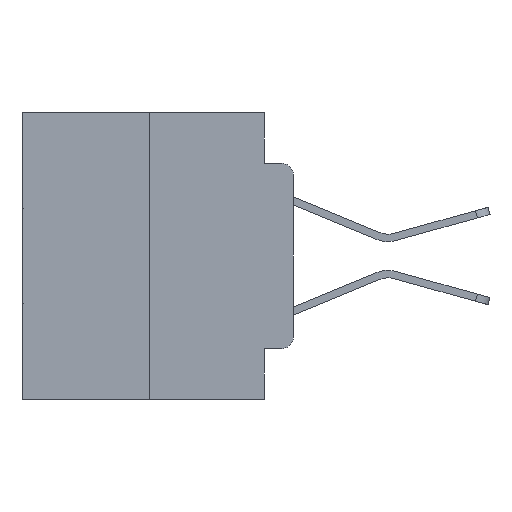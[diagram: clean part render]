
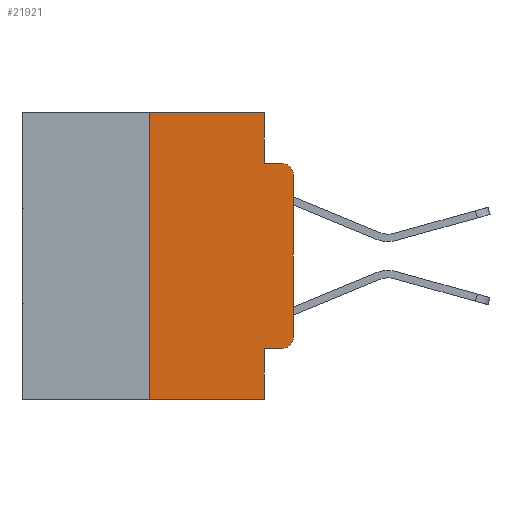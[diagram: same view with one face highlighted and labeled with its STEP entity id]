
A CAD part, left-side view. The second image highlights one B-rep face of the part: STEP entity #21921.
In plain terms, the highlighted planar face has unit normal (-1, 0, 0).
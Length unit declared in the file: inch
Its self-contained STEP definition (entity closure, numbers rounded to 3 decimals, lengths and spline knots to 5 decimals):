
#330 = CARTESIAN_POINT ( 'NONE',  ( 0., 0., -0.1085 ) ) ;
#350 = VECTOR ( 'NONE', #12200, 39.37008 ) ;
#386 = DIRECTION ( 'NONE',  ( 0., 0., -1. ) ) ;
#1704 = DIRECTION ( 'NONE',  ( 0., 0., -1. ) ) ;
#1773 = VECTOR ( 'NONE', #19483, 39.37008 ) ;
#2817 = EDGE_CURVE ( 'NONE', #12098, #9315, #23318, .T. ) ;
#2870 = CARTESIAN_POINT ( 'NONE',  ( 0., 0.473, 0. ) ) ;
#3763 = VECTOR ( 'NONE', #8072, 39.37008 ) ;
#4095 = VERTEX_POINT ( 'NONE', #23252 ) ;
#4832 = ORIENTED_EDGE ( 'NONE', *, *, #26236, .F. ) ;
#4875 = VERTEX_POINT ( 'NONE', #330 ) ;
#5567 = VECTOR ( 'NONE', #23165, 39.37008 ) ;
#5575 = ORIENTED_EDGE ( 'NONE', *, *, #23562, .F. ) ;
#5622 = ORIENTED_EDGE ( 'NONE', *, *, #11684, .T. ) ;
#5971 = DIRECTION ( 'NONE',  ( -1., 0., 0. ) ) ;
#6071 = EDGE_CURVE ( 'NONE', #4095, #27044, #8423, .T. ) ;
#6340 = DIRECTION ( 'NONE',  ( -1., 0., 0. ) ) ;
#6938 = ORIENTED_EDGE ( 'NONE', *, *, #9212, .T. ) ;
#7128 = VERTEX_POINT ( 'NONE', #18365 ) ;
#7258 = CIRCLE ( 'NONE', #7413, 0.02 ) ;
#7413 = AXIS2_PLACEMENT_3D ( 'NONE', #18805, #5971, #20948 ) ;
#8037 = CARTESIAN_POINT ( 'NONE',  ( 0., 0.051, -0.0885 ) ) ;
#8072 = DIRECTION ( 'NONE',  ( 0., -1., 0. ) ) ;
#8423 = LINE ( 'NONE', #21284, #12117 ) ;
#9212 = EDGE_CURVE ( 'NONE', #4875, #13563, #7258, .T. ) ;
#9315 = VERTEX_POINT ( 'NONE', #27440 ) ;
#10048 = CARTESIAN_POINT ( 'NONE',  ( 0., 0.051, -0.4115 ) ) ;
#10429 = CARTESIAN_POINT ( 'NONE',  ( 0., 0.02, -0.0885 ) ) ;
#10655 = ORIENTED_EDGE ( 'NONE', *, *, #6071, .T. ) ;
#11000 = VECTOR ( 'NONE', #13348, 39.37008 ) ;
#11150 = EDGE_CURVE ( 'NONE', #7128, #21916, #21024, .T. ) ;
#11209 = CARTESIAN_POINT ( 'NONE',  ( 0., 0.051, 0. ) ) ;
#11324 = ORIENTED_EDGE ( 'NONE', *, *, #2817, .F. ) ;
#11397 = AXIS2_PLACEMENT_3D ( 'NONE', #19163, #6340, #21306 ) ;
#11595 = CARTESIAN_POINT ( 'NONE',  ( 0., 0.051, -0.4115 ) ) ;
#11684 = EDGE_CURVE ( 'NONE', #21916, #4875, #11994, .T. ) ;
#11979 = LINE ( 'NONE', #26219, #22616 ) ;
#11994 = LINE ( 'NONE', #25247, #5567 ) ;
#12042 = VECTOR ( 'NONE', #20514, 39.37008 ) ;
#12098 = VERTEX_POINT ( 'NONE', #26569 ) ;
#12117 = VECTOR ( 'NONE', #17084, 39.37008 ) ;
#12138 = LINE ( 'NONE', #10048, #350 ) ;
#12200 = DIRECTION ( 'NONE',  ( 0., -1., 0. ) ) ;
#12655 = PLANE ( 'NONE',  #14990 ) ;
#13348 = DIRECTION ( 'NONE',  ( 0., 0., -1. ) ) ;
#13563 = VERTEX_POINT ( 'NONE', #10429 ) ;
#13980 = CARTESIAN_POINT ( 'NONE',  ( 0., 0.051, -0.5 ) ) ;
#14808 = DIRECTION ( 'NONE',  ( 1., 0., 0. ) ) ;
#14983 = ORIENTED_EDGE ( 'NONE', *, *, #20941, .F. ) ;
#14990 = AXIS2_PLACEMENT_3D ( 'NONE', #27368, #14808, #1704 ) ;
#15281 = LINE ( 'NONE', #20758, #3763 ) ;
#15323 = CARTESIAN_POINT ( 'NONE',  ( 0., 0.25, 0. ) ) ;
#17084 = DIRECTION ( 'NONE',  ( 0., -1., 0. ) ) ;
#17808 = VERTEX_POINT ( 'NONE', #8037 ) ;
#17860 = EDGE_LOOP ( 'NONE', ( #5622, #6938, #18990, #5575, #11324, #4832, #10655, #14983, #26830, #19284 ) ) ;
#18365 = CARTESIAN_POINT ( 'NONE',  ( 0., 0.02, -0.4115 ) ) ;
#18805 = CARTESIAN_POINT ( 'NONE',  ( 0., 0.02, -0.1085 ) ) ;
#18939 = EDGE_CURVE ( 'NONE', #26386, #7128, #12138, .T. ) ;
#18990 = ORIENTED_EDGE ( 'NONE', *, *, #23858, .F. ) ;
#19163 = CARTESIAN_POINT ( 'NONE',  ( 0., 0.02, -0.3915 ) ) ;
#19284 = ORIENTED_EDGE ( 'NONE', *, *, #11150, .T. ) ;
#19483 = DIRECTION ( 'NONE',  ( 0., 0., 1. ) ) ;
#20514 = DIRECTION ( 'NONE',  ( 0., -1., 0. ) ) ;
#20758 = CARTESIAN_POINT ( 'NONE',  ( 0., 0.051, -0.0885 ) ) ;
#20941 = EDGE_CURVE ( 'NONE', #26386, #27044, #27762, .T. ) ;
#20948 = DIRECTION ( 'NONE',  ( 0., 0., -1. ) ) ;
#21024 = CIRCLE ( 'NONE', #11397, 0.02 ) ;
#21284 = CARTESIAN_POINT ( 'NONE',  ( 0., 0.473, -0.5 ) ) ;
#21306 = DIRECTION ( 'NONE',  ( 0., 0., -1. ) ) ;
#21916 = VERTEX_POINT ( 'NONE', #25248 ) ;
#21921 = ADVANCED_FACE ( 'NONE', ( #25813 ), #12655, .F. ) ;
#22616 = VECTOR ( 'NONE', #386, 39.37008 ) ;
#23165 = DIRECTION ( 'NONE',  ( 0., 0., 1. ) ) ;
#23252 = CARTESIAN_POINT ( 'NONE',  ( 0., 0.25, -0.5 ) ) ;
#23318 = LINE ( 'NONE', #2870, #12042 ) ;
#23562 = EDGE_CURVE ( 'NONE', #9315, #17808, #11979, .T. ) ;
#23858 = EDGE_CURVE ( 'NONE', #17808, #13563, #15281, .T. ) ;
#24717 = LINE ( 'NONE', #15323, #1773 ) ;
#25247 = CARTESIAN_POINT ( 'NONE',  ( 0., 0., 0. ) ) ;
#25248 = CARTESIAN_POINT ( 'NONE',  ( 0., 0., -0.3915 ) ) ;
#25813 = FACE_OUTER_BOUND ( 'NONE', #17860, .T. ) ;
#26219 = CARTESIAN_POINT ( 'NONE',  ( 0., 0.051, 0. ) ) ;
#26236 = EDGE_CURVE ( 'NONE', #4095, #12098, #24717, .T. ) ;
#26386 = VERTEX_POINT ( 'NONE', #11595 ) ;
#26569 = CARTESIAN_POINT ( 'NONE',  ( 0., 0.25, 0. ) ) ;
#26830 = ORIENTED_EDGE ( 'NONE', *, *, #18939, .T. ) ;
#27044 = VERTEX_POINT ( 'NONE', #13980 ) ;
#27368 = CARTESIAN_POINT ( 'NONE',  ( 0., 0.473, 0. ) ) ;
#27440 = CARTESIAN_POINT ( 'NONE',  ( 0., 0.051, 0. ) ) ;
#27762 = LINE ( 'NONE', #11209, #11000 ) ;
